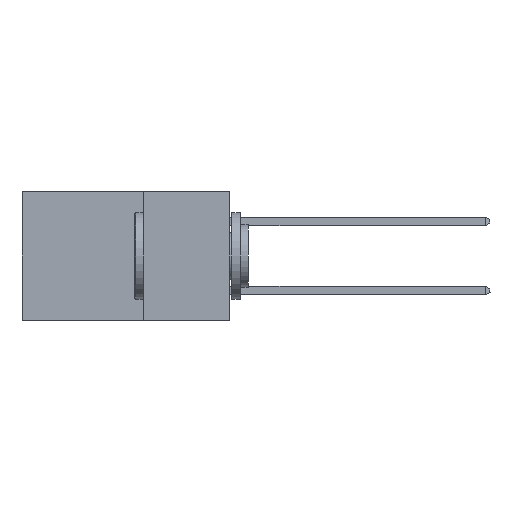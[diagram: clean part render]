
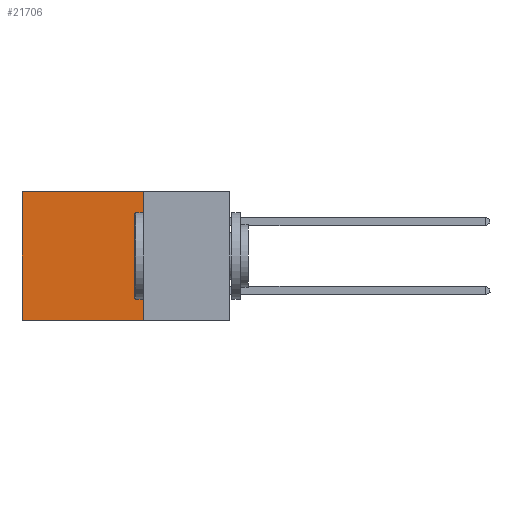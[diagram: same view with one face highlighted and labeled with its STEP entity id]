
A CAD part, left-side view. The second image highlights one B-rep face of the part: STEP entity #21706.
In plain terms, the highlighted planar face has unit normal (-1, 0, 0).
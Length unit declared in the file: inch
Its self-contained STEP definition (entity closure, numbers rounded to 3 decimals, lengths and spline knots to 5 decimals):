
#1474 = VERTEX_POINT ( 'NONE', #13462 ) ;
#1484 = LINE ( 'NONE', #10453, #6415 ) ;
#2428 = VERTEX_POINT ( 'NONE', #18952 ) ;
#2576 = EDGE_CURVE ( 'NONE', #1474, #2428, #14345, .T. ) ;
#2601 = CARTESIAN_POINT ( 'NONE',  ( 0.298, 0.6, 0. ) ) ;
#3241 = ORIENTED_EDGE ( 'NONE', *, *, #10396, .T. ) ;
#3386 = FACE_OUTER_BOUND ( 'NONE', #20732, .T. ) ;
#3865 = VERTEX_POINT ( 'NONE', #23259 ) ;
#4511 = CARTESIAN_POINT ( 'NONE',  ( 0.298, 0.6, 0. ) ) ;
#5581 = LINE ( 'NONE', #4511, #23572 ) ;
#5669 = VECTOR ( 'NONE', #11456, 39.37008 ) ;
#6144 = EDGE_CURVE ( 'NONE', #1474, #13550, #1484, .T. ) ;
#6415 = VECTOR ( 'NONE', #14474, 39.37008 ) ;
#6740 = DIRECTION ( 'NONE',  ( 0., 0., -1. ) ) ;
#9359 = PLANE ( 'NONE',  #10341 ) ;
#10341 = AXIS2_PLACEMENT_3D ( 'NONE', #18938, #23107, #11420 ) ;
#10396 = EDGE_CURVE ( 'NONE', #13550, #3865, #5581, .T. ) ;
#10453 = CARTESIAN_POINT ( 'NONE',  ( 0.298, 0.25, 0. ) ) ;
#10715 = CARTESIAN_POINT ( 'NONE',  ( 0.298, 0.25, 0. ) ) ;
#11420 = DIRECTION ( 'NONE',  ( 0., 0., -1. ) ) ;
#11456 = DIRECTION ( 'NONE',  ( 0., 1., 0. ) ) ;
#13462 = CARTESIAN_POINT ( 'NONE',  ( 0.298, 0.25, 0. ) ) ;
#13550 = VERTEX_POINT ( 'NONE', #2601 ) ;
#14345 = LINE ( 'NONE', #10715, #15550 ) ;
#14474 = DIRECTION ( 'NONE',  ( 0., 1., 0. ) ) ;
#15450 = ORIENTED_EDGE ( 'NONE', *, *, #2576, .F. ) ;
#15550 = VECTOR ( 'NONE', #6740, 39.37008 ) ;
#18309 = DIRECTION ( 'NONE',  ( 0., 0., -1. ) ) ;
#18480 = ORIENTED_EDGE ( 'NONE', *, *, #6144, .T. ) ;
#18938 = CARTESIAN_POINT ( 'NONE',  ( 0.298, 0.25, 0. ) ) ;
#18952 = CARTESIAN_POINT ( 'NONE',  ( 0.298, 0.25, -0.37 ) ) ;
#19234 = CARTESIAN_POINT ( 'NONE',  ( 0.298, 0.25, -0.37 ) ) ;
#19627 = EDGE_CURVE ( 'NONE', #2428, #3865, #21824, .T. ) ;
#20732 = EDGE_LOOP ( 'NONE', ( #3241, #24657, #15450, #18480 ) ) ;
#21706 = ADVANCED_FACE ( 'NONE', ( #3386 ), #9359, .F. ) ;
#21824 = LINE ( 'NONE', #19234, #5669 ) ;
#23107 = DIRECTION ( 'NONE',  ( 1., 0., 0. ) ) ;
#23259 = CARTESIAN_POINT ( 'NONE',  ( 0.298, 0.6, -0.37 ) ) ;
#23572 = VECTOR ( 'NONE', #18309, 39.37008 ) ;
#24657 = ORIENTED_EDGE ( 'NONE', *, *, #19627, .F. ) ;
